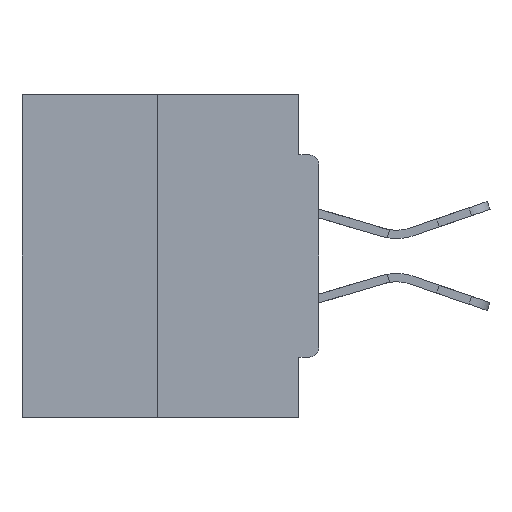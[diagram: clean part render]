
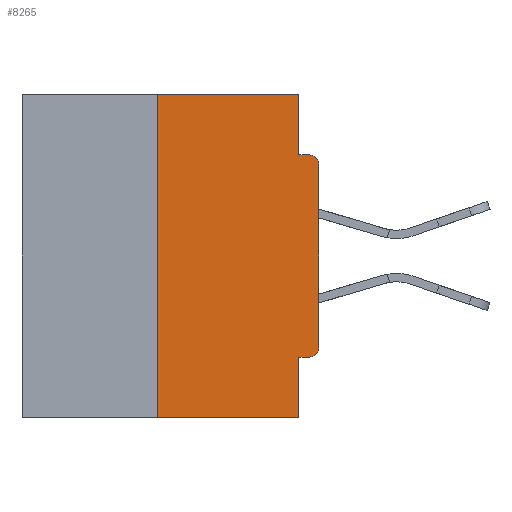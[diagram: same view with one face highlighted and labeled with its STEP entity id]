
A CAD part, left-side view. The second image highlights one B-rep face of the part: STEP entity #8265.
In plain terms, the highlighted planar face has unit normal (-1, 0, 0).
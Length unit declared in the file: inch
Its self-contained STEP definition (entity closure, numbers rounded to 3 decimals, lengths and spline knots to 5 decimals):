
#8 = VERTEX_POINT ( 'NONE', #22056 ) ;
#1129 = DIRECTION ( 'NONE',  ( 0., -1., 0. ) ) ;
#1265 = CARTESIAN_POINT ( 'NONE',  ( 0., 0.031, -0.4065 ) ) ;
#1767 = LINE ( 'NONE', #13883, #2705 ) ;
#1872 = VERTEX_POINT ( 'NONE', #22339 ) ;
#2287 = ORIENTED_EDGE ( 'NONE', *, *, #20171, .F. ) ;
#2315 = LINE ( 'NONE', #37241, #34627 ) ;
#2705 = VECTOR ( 'NONE', #14153, 39.37008 ) ;
#2739 = LINE ( 'NONE', #13316, #25063 ) ;
#3029 = DIRECTION ( 'NONE',  ( 0., 1., 0. ) ) ;
#3155 = VERTEX_POINT ( 'NONE', #5794 ) ;
#3719 = CARTESIAN_POINT ( 'NONE',  ( 0., 0.031, -0.5 ) ) ;
#4362 = ORIENTED_EDGE ( 'NONE', *, *, #18404, .T. ) ;
#5151 = ORIENTED_EDGE ( 'NONE', *, *, #33347, .F. ) ;
#5794 = CARTESIAN_POINT ( 'NONE',  ( 0., 0., -0.3915 ) ) ;
#6654 = EDGE_LOOP ( 'NONE', ( #12045, #36474, #30046, #5151, #28998, #4362, #38168, #30384, #37215, #2287 ) ) ;
#7674 = FACE_OUTER_BOUND ( 'NONE', #6654, .T. ) ;
#8265 = ADVANCED_FACE ( 'NONE', ( #7674 ), #14011, .F. ) ;
#9404 = DIRECTION ( 'NONE',  ( 0., 0., -1. ) ) ;
#9952 = CARTESIAN_POINT ( 'NONE',  ( 0., 0.015, -0.4065 ) ) ;
#11560 = CARTESIAN_POINT ( 'NONE',  ( 0., 0.031, -0.0935 ) ) ;
#12031 = AXIS2_PLACEMENT_3D ( 'NONE', #25380, #34692, #37766 ) ;
#12045 = ORIENTED_EDGE ( 'NONE', *, *, #28352, .F. ) ;
#13316 = CARTESIAN_POINT ( 'NONE',  ( 0., 0.46, 0. ) ) ;
#13618 = CARTESIAN_POINT ( 'NONE',  ( 0., 0., 0. ) ) ;
#13866 = VECTOR ( 'NONE', #31223, 39.37008 ) ;
#13883 = CARTESIAN_POINT ( 'NONE',  ( 0., 0.031, 0. ) ) ;
#14011 = PLANE ( 'NONE',  #34294 ) ;
#14153 = DIRECTION ( 'NONE',  ( 0., 0., -1. ) ) ;
#15708 = VERTEX_POINT ( 'NONE', #36691 ) ;
#16022 = DIRECTION ( 'NONE',  ( 0., 0., 1. ) ) ;
#16744 = LINE ( 'NONE', #3719, #13866 ) ;
#17656 = VECTOR ( 'NONE', #3029, 39.37008 ) ;
#17705 = EDGE_CURVE ( 'NONE', #19080, #38516, #38575, .T. ) ;
#18399 = VECTOR ( 'NONE', #16022, 39.37008 ) ;
#18404 = EDGE_CURVE ( 'NONE', #19080, #3155, #32325, .T. ) ;
#18420 = CARTESIAN_POINT ( 'NONE',  ( 0., 0.015, -0.3915 ) ) ;
#18426 = AXIS2_PLACEMENT_3D ( 'NONE', #18420, #21727, #9404 ) ;
#19022 = DIRECTION ( 'NONE',  ( 0., -1., 0. ) ) ;
#19080 = VERTEX_POINT ( 'NONE', #9952 ) ;
#19731 = DIRECTION ( 'NONE',  ( 0., 0., 1. ) ) ;
#20171 = EDGE_CURVE ( 'NONE', #20627, #37332, #1767, .T. ) ;
#20627 = VERTEX_POINT ( 'NONE', #34968 ) ;
#21179 = LINE ( 'NONE', #39278, #39301 ) ;
#21468 = CARTESIAN_POINT ( 'NONE',  ( 0., 0., -0.1085 ) ) ;
#21727 = DIRECTION ( 'NONE',  ( -1., 0., 0. ) ) ;
#22056 = CARTESIAN_POINT ( 'NONE',  ( 0., 0.25, -0.5 ) ) ;
#22328 = EDGE_CURVE ( 'NONE', #8, #1872, #35022, .T. ) ;
#22339 = CARTESIAN_POINT ( 'NONE',  ( 0., 0.25, 0. ) ) ;
#22903 = CARTESIAN_POINT ( 'NONE',  ( 0., 0.46, 0. ) ) ;
#25063 = VECTOR ( 'NONE', #1129, 39.37008 ) ;
#25380 = CARTESIAN_POINT ( 'NONE',  ( 0., 0.015, -0.1085 ) ) ;
#26383 = VECTOR ( 'NONE', #19731, 39.37008 ) ;
#27136 = DIRECTION ( 'NONE',  ( 0., -1., 0. ) ) ;
#28352 = EDGE_CURVE ( 'NONE', #1872, #20627, #2739, .T. ) ;
#28998 = ORIENTED_EDGE ( 'NONE', *, *, #17705, .F. ) ;
#30046 = ORIENTED_EDGE ( 'NONE', *, *, #30749, .T. ) ;
#30081 = DIRECTION ( 'NONE',  ( 0., 0., -1. ) ) ;
#30113 = VERTEX_POINT ( 'NONE', #35701 ) ;
#30384 = ORIENTED_EDGE ( 'NONE', *, *, #35930, .T. ) ;
#30662 = LINE ( 'NONE', #13618, #26383 ) ;
#30749 = EDGE_CURVE ( 'NONE', #8, #30113, #21179, .T. ) ;
#31223 = DIRECTION ( 'NONE',  ( 0., 0., -1. ) ) ;
#32325 = CIRCLE ( 'NONE', #18426, 0.015 ) ;
#33347 = EDGE_CURVE ( 'NONE', #38516, #30113, #16744, .T. ) ;
#34101 = CARTESIAN_POINT ( 'NONE',  ( 0., 0.25, 0. ) ) ;
#34294 = AXIS2_PLACEMENT_3D ( 'NONE', #22903, #35666, #30081 ) ;
#34627 = VECTOR ( 'NONE', #19022, 39.37008 ) ;
#34692 = DIRECTION ( 'NONE',  ( -1., 0., 0. ) ) ;
#34968 = CARTESIAN_POINT ( 'NONE',  ( 0., 0.031, 0. ) ) ;
#35022 = LINE ( 'NONE', #34101, #18399 ) ;
#35666 = DIRECTION ( 'NONE',  ( 1., 0., 0. ) ) ;
#35701 = CARTESIAN_POINT ( 'NONE',  ( 0., 0.031, -0.5 ) ) ;
#35803 = EDGE_CURVE ( 'NONE', #37332, #15708, #2315, .T. ) ;
#35930 = EDGE_CURVE ( 'NONE', #36822, #15708, #38925, .T. ) ;
#36362 = CARTESIAN_POINT ( 'NONE',  ( 0., 0., -0.4065 ) ) ;
#36474 = ORIENTED_EDGE ( 'NONE', *, *, #22328, .F. ) ;
#36691 = CARTESIAN_POINT ( 'NONE',  ( 0., 0.015, -0.0935 ) ) ;
#36822 = VERTEX_POINT ( 'NONE', #21468 ) ;
#37092 = EDGE_CURVE ( 'NONE', #3155, #36822, #30662, .T. ) ;
#37215 = ORIENTED_EDGE ( 'NONE', *, *, #35803, .F. ) ;
#37241 = CARTESIAN_POINT ( 'NONE',  ( 0., 0., -0.0935 ) ) ;
#37332 = VERTEX_POINT ( 'NONE', #11560 ) ;
#37766 = DIRECTION ( 'NONE',  ( 0., 0., -1. ) ) ;
#38168 = ORIENTED_EDGE ( 'NONE', *, *, #37092, .T. ) ;
#38516 = VERTEX_POINT ( 'NONE', #1265 ) ;
#38575 = LINE ( 'NONE', #36362, #17656 ) ;
#38925 = CIRCLE ( 'NONE', #12031, 0.015 ) ;
#39278 = CARTESIAN_POINT ( 'NONE',  ( 0., 0.46, -0.5 ) ) ;
#39301 = VECTOR ( 'NONE', #27136, 39.37008 ) ;
